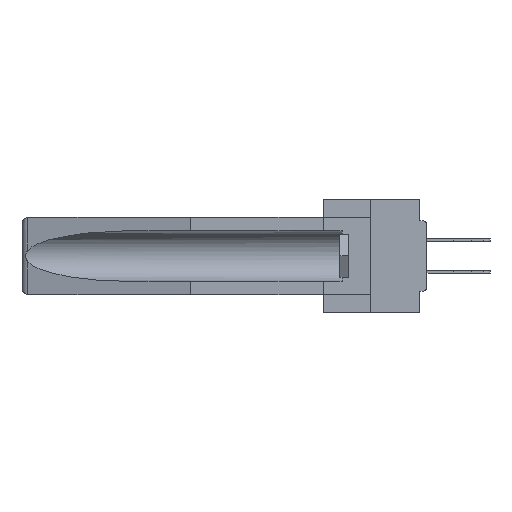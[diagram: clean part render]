
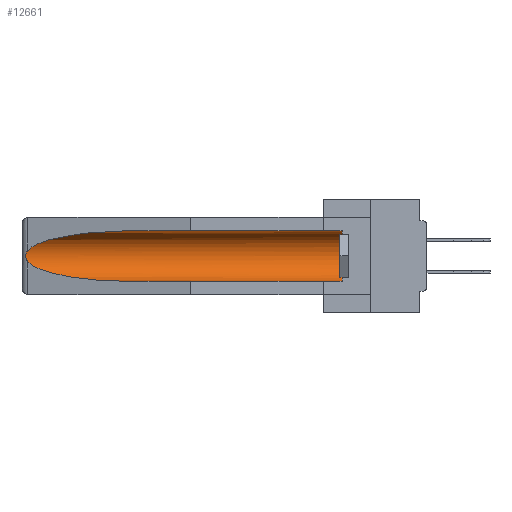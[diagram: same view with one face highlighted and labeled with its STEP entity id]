
A CAD part, left-side view. The second image highlights one B-rep face of the part: STEP entity #12661.
In plain terms, the highlighted cylindrical face has radius 2.857 mm (diameter 5.715 mm), a partial arc.
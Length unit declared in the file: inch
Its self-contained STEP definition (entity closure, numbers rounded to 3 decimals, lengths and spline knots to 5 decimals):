
#836 = EDGE_CURVE ( 'NONE', #17018, #26817, #29346, .T. ) ;
#1124 = CARTESIAN_POINT ( 'NONE',  ( 0.21114, 1.30732, -0.284 ) ) ;
#1303 = CARTESIAN_POINT ( 'NONE',  ( 0.26654, 1.53092, -0.15636 ) ) ;
#2418 =( BOUNDED_CURVE ( )  B_SPLINE_CURVE ( 3, ( #31114, #3881, #1124, #3537 ),
 .UNSPECIFIED., .F., .F. ) 
 B_SPLINE_CURVE_WITH_KNOTS ( ( 4, 4 ),
 ( 0.1948, 1.5708 ),
 .UNSPECIFIED. ) 
 CURVE ( )  GEOMETRIC_REPRESENTATION_ITEM ( )  RATIONAL_B_SPLINE_CURVE ( ( 1., 0.848, 0.848, 1. ) ) 
 REPRESENTATION_ITEM ( '' )  );
#3388 = CIRCLE ( 'NONE', #5835, 0.1125 ) ;
#3537 = CARTESIAN_POINT ( 'NONE',  ( 0.155, 1.07973, -0.284 ) ) ;
#3822 = CARTESIAN_POINT ( 'NONE',  ( 0.2675, 1.53308, -0.17534 ) ) ;
#3881 = CARTESIAN_POINT ( 'NONE',  ( 0.25451, 1.48313, -0.24835 ) ) ;
#3937 = CARTESIAN_POINT ( 'NONE',  ( 0.26537, 1.52718, -0.14972 ) ) ;
#4285 = CARTESIAN_POINT ( 'NONE',  ( 0.155, -0.30754, -0.284 ) ) ;
#4395 =( BOUNDED_CURVE ( )  B_SPLINE_CURVE ( 3, ( #15017, #18604, #31983, #4520 ),
 .UNSPECIFIED., .F., .F. ) 
 B_SPLINE_CURVE_WITH_KNOTS ( ( 4, 4 ),
 ( 4.71239, 6.08839 ),
 .UNSPECIFIED. ) 
 CURVE ( )  GEOMETRIC_REPRESENTATION_ITEM ( )  RATIONAL_B_SPLINE_CURVE ( ( 1., 0.848, 0.848, 1. ) ) 
 REPRESENTATION_ITEM ( '' )  );
#4520 = CARTESIAN_POINT ( 'NONE',  ( 0.26537, 1.52718, -0.14972 ) ) ;
#4588 = AXIS2_PLACEMENT_3D ( 'NONE', #33869, #25602, #14585 ) ;
#4775 = ORIENTED_EDGE ( 'NONE', *, *, #32869, .T. ) ;
#5510 = VERTEX_POINT ( 'NONE', #35326 ) ;
#5596 = FACE_OUTER_BOUND ( 'NONE', #9268, .T. ) ;
#5835 = AXIS2_PLACEMENT_3D ( 'NONE', #29912, #13513, #35427 ) ;
#6717 = VECTOR ( 'NONE', #29703, 39.37008 ) ;
#6804 = EDGE_CURVE ( 'NONE', #19250, #5510, #3388, .T. ) ;
#9268 = EDGE_LOOP ( 'NONE', ( #4775, #34181, #22515, #10611, #33520, #29008 ) ) ;
#10611 = ORIENTED_EDGE ( 'NONE', *, *, #32686, .F. ) ;
#10967 = LINE ( 'NONE', #35441, #6717 ) ;
#11067 = CARTESIAN_POINT ( 'NONE',  ( 0.26537, 1.52718, -0.14972 ) ) ;
#11118 = CYLINDRICAL_SURFACE ( 'NONE', #4588, 0.1125 ) ;
#12371 = CARTESIAN_POINT ( 'NONE',  ( 0.2673, 1.5327, -0.16383 ) ) ;
#12661 = ADVANCED_FACE ( 'NONE', ( #5596 ), #11118, .F. ) ;
#12708 = LINE ( 'NONE', #4285, #29404 ) ;
#13313 = CARTESIAN_POINT ( 'NONE',  ( 0.26537, 1.52718, -0.19328 ) ) ;
#13513 = DIRECTION ( 'NONE',  ( 0., -1., 0. ) ) ;
#14585 = DIRECTION ( 'NONE',  ( 0., 0., 1. ) ) ;
#15017 = CARTESIAN_POINT ( 'NONE',  ( 0.155, 1.07973, -0.059 ) ) ;
#17018 = VERTEX_POINT ( 'NONE', #11067 ) ;
#17595 = CARTESIAN_POINT ( 'NONE',  ( 0.155, 0.126, -0.284 ) ) ;
#18604 = CARTESIAN_POINT ( 'NONE',  ( 0.21114, 1.30732, -0.059 ) ) ;
#19250 = VERTEX_POINT ( 'NONE', #17595 ) ;
#22042 = VERTEX_POINT ( 'NONE', #33222 ) ;
#22515 = ORIENTED_EDGE ( 'NONE', *, *, #33335, .T. ) ;
#22963 = CARTESIAN_POINT ( 'NONE',  ( 0.26597, 1.5296, -0.19026 ) ) ;
#23074 = CARTESIAN_POINT ( 'NONE',  ( 0.2673, 1.53269, -0.17917 ) ) ;
#23417 = DIRECTION ( 'NONE',  ( 0., 1., 0. ) ) ;
#25602 = DIRECTION ( 'NONE',  ( 0., 1., 0. ) ) ;
#26145 = CARTESIAN_POINT ( 'NONE',  ( 0.26597, 1.52961, -0.15275 ) ) ;
#26817 = VERTEX_POINT ( 'NONE', #13313 ) ;
#27363 = CARTESIAN_POINT ( 'NONE',  ( 0.155, 1.07973, -0.059 ) ) ;
#28426 = CARTESIAN_POINT ( 'NONE',  ( 0.2675, 1.53308, -0.16763 ) ) ;
#29008 = ORIENTED_EDGE ( 'NONE', *, *, #33052, .T. ) ;
#29151 = VERTEX_POINT ( 'NONE', #27363 ) ;
#29346 = B_SPLINE_CURVE_WITH_KNOTS ( 'NONE', 3,
 ( #3937, #26145, #1303, #12371, #28426, #3822, #23074, #31532, #22963, #33968 ),
 .UNSPECIFIED., .F., .F.,
 ( 4, 2, 2, 2, 4 ),
 ( 0., 0.00029, 0.00058, 0.00087, 0.00117 ),
 .UNSPECIFIED. ) ;
#29404 = VECTOR ( 'NONE', #23417, 39.37008 ) ;
#29703 = DIRECTION ( 'NONE',  ( 0., 1., 0. ) ) ;
#29912 = CARTESIAN_POINT ( 'NONE',  ( 0.155, 0.126, -0.1715 ) ) ;
#31114 = CARTESIAN_POINT ( 'NONE',  ( 0.26537, 1.52718, -0.19328 ) ) ;
#31532 = CARTESIAN_POINT ( 'NONE',  ( 0.26655, 1.53094, -0.18657 ) ) ;
#31983 = CARTESIAN_POINT ( 'NONE',  ( 0.25451, 1.48313, -0.09465 ) ) ;
#32686 = EDGE_CURVE ( 'NONE', #19250, #22042, #12708, .T. ) ;
#32869 = EDGE_CURVE ( 'NONE', #29151, #17018, #4395, .T. ) ;
#33052 = EDGE_CURVE ( 'NONE', #5510, #29151, #10967, .T. ) ;
#33222 = CARTESIAN_POINT ( 'NONE',  ( 0.155, 1.07973, -0.284 ) ) ;
#33335 = EDGE_CURVE ( 'NONE', #26817, #22042, #2418, .T. ) ;
#33520 = ORIENTED_EDGE ( 'NONE', *, *, #6804, .T. ) ;
#33869 = CARTESIAN_POINT ( 'NONE',  ( 0.155, -0.30754, -0.1715 ) ) ;
#33968 = CARTESIAN_POINT ( 'NONE',  ( 0.26537, 1.52718, -0.19328 ) ) ;
#34181 = ORIENTED_EDGE ( 'NONE', *, *, #836, .T. ) ;
#35326 = CARTESIAN_POINT ( 'NONE',  ( 0.155, 0.126, -0.059 ) ) ;
#35427 = DIRECTION ( 'NONE',  ( 0., 0., 1. ) ) ;
#35441 = CARTESIAN_POINT ( 'NONE',  ( 0.155, -0.30754, -0.059 ) ) ;
